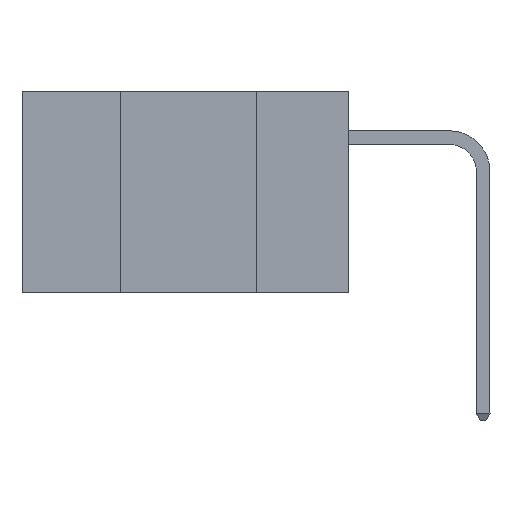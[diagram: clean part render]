
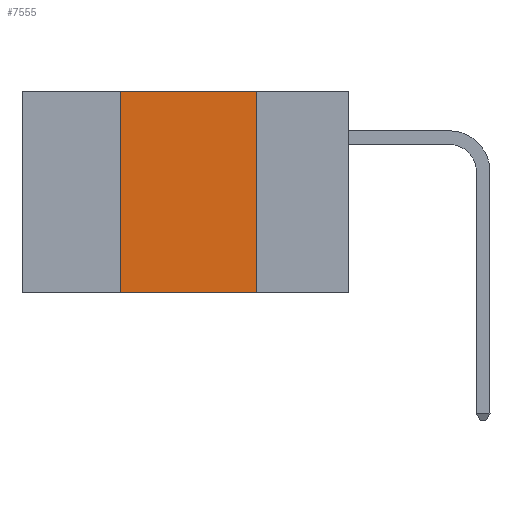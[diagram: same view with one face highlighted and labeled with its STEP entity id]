
A CAD part, left-side view. The second image highlights one B-rep face of the part: STEP entity #7555.
In plain terms, the highlighted planar face has unit normal (-1, 0, 0).
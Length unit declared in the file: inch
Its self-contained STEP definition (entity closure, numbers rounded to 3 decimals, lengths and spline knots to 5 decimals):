
#194 = ORIENTED_EDGE ( 'NONE', *, *, #6080, .F. ) ;
#395 = VERTEX_POINT ( 'NONE', #6368 ) ;
#447 = CARTESIAN_POINT ( 'NONE',  ( 0., 0.42, 0. ) ) ;
#1022 = LINE ( 'NONE', #9200, #3566 ) ;
#1404 = LINE ( 'NONE', #447, #2615 ) ;
#1844 = DIRECTION ( 'NONE',  ( 0., -1., 0. ) ) ;
#1857 = CARTESIAN_POINT ( 'NONE',  ( 0., 0.42, 0. ) ) ;
#1901 = LINE ( 'NONE', #2774, #4701 ) ;
#2134 = VECTOR ( 'NONE', #8482, 39.37008 ) ;
#2350 = PLANE ( 'NONE',  #4379 ) ;
#2609 = EDGE_CURVE ( 'NONE', #7040, #8808, #1022, .T. ) ;
#2615 = VECTOR ( 'NONE', #9578, 39.37008 ) ;
#2666 = DIRECTION ( 'NONE',  ( 0., -1., 0. ) ) ;
#2774 = CARTESIAN_POINT ( 'NONE',  ( 0., 0.6, 0. ) ) ;
#3566 = VECTOR ( 'NONE', #1844, 39.37008 ) ;
#3590 = EDGE_CURVE ( 'NONE', #7040, #9532, #1404, .T. ) ;
#3668 = LINE ( 'NONE', #6721, #2134 ) ;
#4254 = ORIENTED_EDGE ( 'NONE', *, *, #6866, .F. ) ;
#4379 = AXIS2_PLACEMENT_3D ( 'NONE', #5649, #9931, #7515 ) ;
#4701 = VECTOR ( 'NONE', #2666, 39.37008 ) ;
#5649 = CARTESIAN_POINT ( 'NONE',  ( 0., 0.6, 0. ) ) ;
#6029 = ORIENTED_EDGE ( 'NONE', *, *, #2609, .T. ) ;
#6080 = EDGE_CURVE ( 'NONE', #395, #8808, #3668, .T. ) ;
#6316 = EDGE_LOOP ( 'NONE', ( #194, #4254, #10398, #6029 ) ) ;
#6368 = CARTESIAN_POINT ( 'NONE',  ( 0., 0.17, 0. ) ) ;
#6721 = CARTESIAN_POINT ( 'NONE',  ( 0., 0.17, 0. ) ) ;
#6866 = EDGE_CURVE ( 'NONE', #9532, #395, #1901, .T. ) ;
#6999 = CARTESIAN_POINT ( 'NONE',  ( 0., 0.17, -0.37 ) ) ;
#7040 = VERTEX_POINT ( 'NONE', #7866 ) ;
#7515 = DIRECTION ( 'NONE',  ( 0., 0., -1. ) ) ;
#7555 = ADVANCED_FACE ( 'NONE', ( #10576 ), #2350, .F. ) ;
#7866 = CARTESIAN_POINT ( 'NONE',  ( 0., 0.42, -0.37 ) ) ;
#8482 = DIRECTION ( 'NONE',  ( 0., 0., -1. ) ) ;
#8808 = VERTEX_POINT ( 'NONE', #6999 ) ;
#9200 = CARTESIAN_POINT ( 'NONE',  ( 0., 0.6, -0.37 ) ) ;
#9532 = VERTEX_POINT ( 'NONE', #1857 ) ;
#9578 = DIRECTION ( 'NONE',  ( 0., 0., 1. ) ) ;
#9931 = DIRECTION ( 'NONE',  ( 1., 0., 0. ) ) ;
#10398 = ORIENTED_EDGE ( 'NONE', *, *, #3590, .F. ) ;
#10576 = FACE_OUTER_BOUND ( 'NONE', #6316, .T. ) ;
